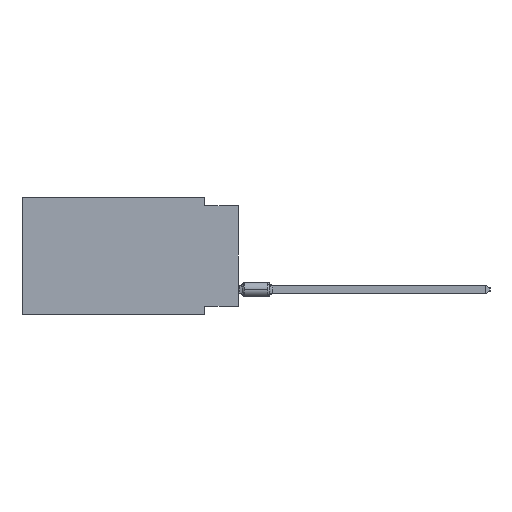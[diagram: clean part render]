
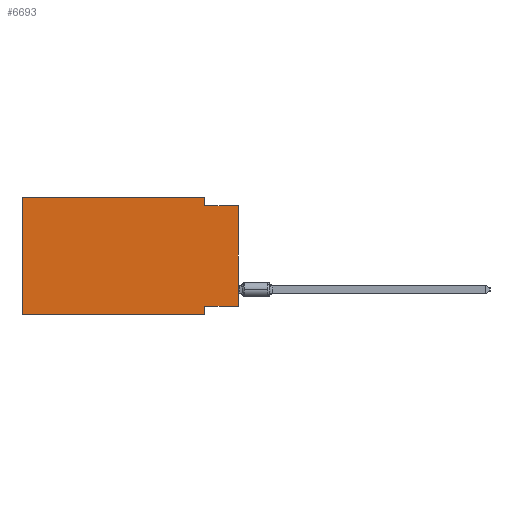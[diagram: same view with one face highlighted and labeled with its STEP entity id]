
A CAD part, left-side view. The second image highlights one B-rep face of the part: STEP entity #6693.
In plain terms, the highlighted planar face has unit normal (-1, 0, 0).
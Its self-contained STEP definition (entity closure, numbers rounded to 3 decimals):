
#1106 = DIRECTION ( 'NONE',  ( 0., -1., 0. ) ) ;
#1545 = DIRECTION ( 'NONE',  ( 0., 0., -1. ) ) ;
#2801 = DIRECTION ( 'NONE',  ( 0., 1., 0. ) ) ;
#3242 = CARTESIAN_POINT ( 'NONE',  ( 0., 2.54, -8.89 ) ) ;
#3607 = ORIENTED_EDGE ( 'NONE', *, *, #19411, .F. ) ;
#3974 = CARTESIAN_POINT ( 'NONE',  ( 0., 16.383, -8.89 ) ) ;
#4811 = VERTEX_POINT ( 'NONE', #31168 ) ;
#4989 = LINE ( 'NONE', #3974, #47841 ) ;
#6165 = VERTEX_POINT ( 'NONE', #38228 ) ;
#6693 = ADVANCED_FACE ( 'NONE', ( #19042 ), #7583, .F. ) ;
#7583 = PLANE ( 'NONE',  #23000 ) ;
#8425 = ORIENTED_EDGE ( 'NONE', *, *, #13410, .F. ) ;
#8639 = EDGE_CURVE ( 'NONE', #29965, #6165, #28333, .T. ) ;
#9038 = CARTESIAN_POINT ( 'NONE',  ( 0., 2.54, 0. ) ) ;
#12001 = DIRECTION ( 'NONE',  ( 1., 0., 0. ) ) ;
#12110 = DIRECTION ( 'NONE',  ( 0., -1., 0. ) ) ;
#13119 = VERTEX_POINT ( 'NONE', #28467 ) ;
#13410 = EDGE_CURVE ( 'NONE', #13119, #6165, #36627, .T. ) ;
#14881 = ORIENTED_EDGE ( 'NONE', *, *, #44119, .T. ) ;
#15100 = ORIENTED_EDGE ( 'NONE', *, *, #28647, .F. ) ;
#15420 = ORIENTED_EDGE ( 'NONE', *, *, #35819, .F. ) ;
#15702 = VERTEX_POINT ( 'NONE', #21103 ) ;
#16010 = CARTESIAN_POINT ( 'NONE',  ( 0., 16.383, 0. ) ) ;
#16187 = CARTESIAN_POINT ( 'NONE',  ( 0., 0., 0. ) ) ;
#18897 = CARTESIAN_POINT ( 'NONE',  ( 0., 16.383, 0. ) ) ;
#19042 = FACE_OUTER_BOUND ( 'NONE', #27711, .T. ) ;
#19330 = DIRECTION ( 'NONE',  ( 0., 0., -1. ) ) ;
#19411 = EDGE_CURVE ( 'NONE', #29420, #15702, #26828, .T. ) ;
#21103 = CARTESIAN_POINT ( 'NONE',  ( 0., 2.54, -8.89 ) ) ;
#23000 = AXIS2_PLACEMENT_3D ( 'NONE', #46702, #12001, #42821 ) ;
#25070 = CARTESIAN_POINT ( 'NONE',  ( 0., 0., -8.255 ) ) ;
#26153 = LINE ( 'NONE', #33913, #27930 ) ;
#26202 = ORIENTED_EDGE ( 'NONE', *, *, #8639, .T. ) ;
#26646 = LINE ( 'NONE', #18897, #30860 ) ;
#26828 = LINE ( 'NONE', #3242, #41099 ) ;
#27711 = EDGE_LOOP ( 'NONE', ( #26202, #8425, #15420, #43348, #15100, #14881, #3607, #33481 ) ) ;
#27930 = VECTOR ( 'NONE', #2801, 1000. ) ;
#28158 = VECTOR ( 'NONE', #12110, 1000. ) ;
#28333 = LINE ( 'NONE', #16187, #42867 ) ;
#28467 = CARTESIAN_POINT ( 'NONE',  ( 0., 2.54, -0.635 ) ) ;
#28647 = EDGE_CURVE ( 'NONE', #42252, #4811, #26646, .T. ) ;
#29420 = VERTEX_POINT ( 'NONE', #38886 ) ;
#29965 = VERTEX_POINT ( 'NONE', #25070 ) ;
#30860 = VECTOR ( 'NONE', #34675, 1000. ) ;
#31168 = CARTESIAN_POINT ( 'NONE',  ( 0., 16.383, 0. ) ) ;
#31971 = DIRECTION ( 'NONE',  ( 0., 0., 1. ) ) ;
#33481 = ORIENTED_EDGE ( 'NONE', *, *, #35899, .F. ) ;
#33757 = VECTOR ( 'NONE', #1545, 1000. ) ;
#33913 = CARTESIAN_POINT ( 'NONE',  ( 0., 0., -8.255 ) ) ;
#34675 = DIRECTION ( 'NONE',  ( 0., 0., 1. ) ) ;
#35813 = VECTOR ( 'NONE', #36111, 1000. ) ;
#35819 = EDGE_CURVE ( 'NONE', #41749, #13119, #37025, .T. ) ;
#35899 = EDGE_CURVE ( 'NONE', #29965, #29420, #26153, .T. ) ;
#36111 = DIRECTION ( 'NONE',  ( 0., -1., 0. ) ) ;
#36627 = LINE ( 'NONE', #39747, #35813 ) ;
#36800 = EDGE_CURVE ( 'NONE', #4811, #41749, #40319, .T. ) ;
#37025 = LINE ( 'NONE', #9038, #33757 ) ;
#38228 = CARTESIAN_POINT ( 'NONE',  ( 0., 0., -0.635 ) ) ;
#38886 = CARTESIAN_POINT ( 'NONE',  ( 0., 2.54, -8.255 ) ) ;
#39747 = CARTESIAN_POINT ( 'NONE',  ( 0., 0., -0.635 ) ) ;
#39748 = CARTESIAN_POINT ( 'NONE',  ( 0., 16.383, -8.89 ) ) ;
#40319 = LINE ( 'NONE', #16010, #28158 ) ;
#41099 = VECTOR ( 'NONE', #19330, 1000. ) ;
#41749 = VERTEX_POINT ( 'NONE', #43686 ) ;
#42252 = VERTEX_POINT ( 'NONE', #39748 ) ;
#42821 = DIRECTION ( 'NONE',  ( 0., 0., -1. ) ) ;
#42867 = VECTOR ( 'NONE', #31971, 1000. ) ;
#43348 = ORIENTED_EDGE ( 'NONE', *, *, #36800, .F. ) ;
#43686 = CARTESIAN_POINT ( 'NONE',  ( 0., 2.54, 0. ) ) ;
#44119 = EDGE_CURVE ( 'NONE', #42252, #15702, #4989, .T. ) ;
#46702 = CARTESIAN_POINT ( 'NONE',  ( 0., 16.383, 0. ) ) ;
#47841 = VECTOR ( 'NONE', #1106, 1000. ) ;
